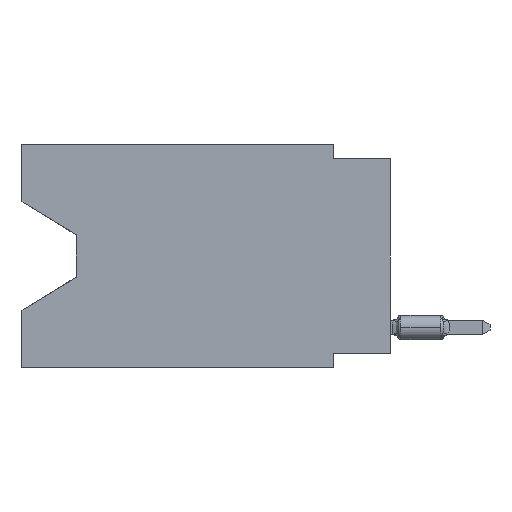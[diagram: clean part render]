
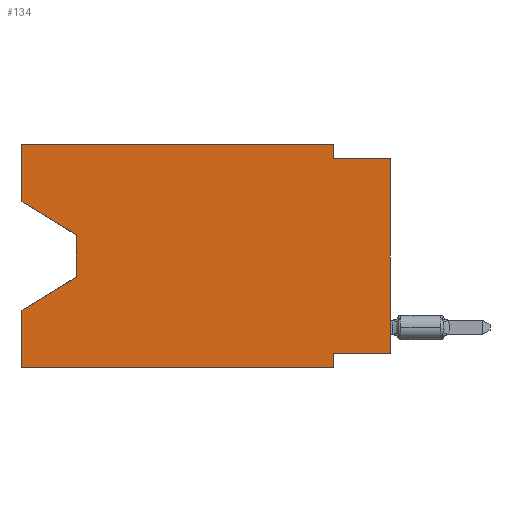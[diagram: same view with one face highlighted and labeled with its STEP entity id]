
A CAD part, left-side view. The second image highlights one B-rep face of the part: STEP entity #134.
In plain terms, the highlighted planar face has unit normal (-1, 0, 0).
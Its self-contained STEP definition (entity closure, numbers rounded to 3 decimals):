
#134 = ADVANCED_FACE ( 'NONE', ( #10927 ), #3493, .F. ) ;
#347 = LINE ( 'NONE', #12735, #4989 ) ;
#407 = LINE ( 'NONE', #6178, #16568 ) ;
#607 = CARTESIAN_POINT ( 'NONE',  ( 0., 2.54, -0.635 ) ) ;
#656 = VECTOR ( 'NONE', #1703, 1000. ) ;
#1014 = CARTESIAN_POINT ( 'NONE',  ( 0., 13.97, -4.013 ) ) ;
#1512 = LINE ( 'NONE', #7038, #6658 ) ;
#1613 = CARTESIAN_POINT ( 'NONE',  ( 0., 16.383, -2.546 ) ) ;
#1703 = DIRECTION ( 'NONE',  ( 0., -1., 0. ) ) ;
#2876 = EDGE_CURVE ( 'NONE', #12312, #13127, #347, .T. ) ;
#3388 = VECTOR ( 'NONE', #4593, 1000. ) ;
#3493 = PLANE ( 'NONE',  #19131 ) ;
#3496 = VERTEX_POINT ( 'NONE', #12833 ) ;
#3534 = ORIENTED_EDGE ( 'NONE', *, *, #12968, .F. ) ;
#3618 = CARTESIAN_POINT ( 'NONE',  ( 0., 16.383, 0. ) ) ;
#3664 = ORIENTED_EDGE ( 'NONE', *, *, #5299, .F. ) ;
#3716 = DIRECTION ( 'NONE',  ( 0., 0., -1. ) ) ;
#3749 = VERTEX_POINT ( 'NONE', #14147 ) ;
#3884 = LINE ( 'NONE', #1613, #22900 ) ;
#3914 = DIRECTION ( 'NONE',  ( 0., 1., 0. ) ) ;
#3937 = EDGE_CURVE ( 'NONE', #19255, #10933, #11486, .T. ) ;
#4223 = CARTESIAN_POINT ( 'NONE',  ( 0., 2.54, -9.906 ) ) ;
#4327 = CARTESIAN_POINT ( 'NONE',  ( 0., 16.383, -2.546 ) ) ;
#4554 = VERTEX_POINT ( 'NONE', #8674 ) ;
#4593 = DIRECTION ( 'NONE',  ( 0., -1., 0. ) ) ;
#4989 = VECTOR ( 'NONE', #3716, 1000. ) ;
#5181 = LINE ( 'NONE', #17962, #12593 ) ;
#5299 = EDGE_CURVE ( 'NONE', #13127, #3749, #19001, .T. ) ;
#6178 = CARTESIAN_POINT ( 'NONE',  ( 0., 16.383, 0. ) ) ;
#6658 = VECTOR ( 'NONE', #21821, 1000. ) ;
#6997 = DIRECTION ( 'NONE',  ( 0., 0., 1. ) ) ;
#7000 = LINE ( 'NONE', #3618, #656 ) ;
#7038 = CARTESIAN_POINT ( 'NONE',  ( 0., 2.54, -9.906 ) ) ;
#7226 = VECTOR ( 'NONE', #3914, 1000. ) ;
#7265 = DIRECTION ( 'NONE',  ( 0., -0.855, -0.519 ) ) ;
#7626 = ORIENTED_EDGE ( 'NONE', *, *, #13353, .T. ) ;
#7737 = DIRECTION ( 'NONE',  ( 0., 0., 1. ) ) ;
#7850 = EDGE_CURVE ( 'NONE', #10156, #19255, #3884, .T. ) ;
#7934 = CARTESIAN_POINT ( 'NONE',  ( 0., 13.97, -5.893 ) ) ;
#8460 = ORIENTED_EDGE ( 'NONE', *, *, #11576, .T. ) ;
#8525 = CARTESIAN_POINT ( 'NONE',  ( 0., 13.97, -5.893 ) ) ;
#8674 = CARTESIAN_POINT ( 'NONE',  ( 0., 16.383, -9.906 ) ) ;
#8904 = ORIENTED_EDGE ( 'NONE', *, *, #2876, .F. ) ;
#9022 = CARTESIAN_POINT ( 'NONE',  ( 0., 16.383, 0. ) ) ;
#9050 = EDGE_CURVE ( 'NONE', #20871, #3749, #5181, .T. ) ;
#9138 = DIRECTION ( 'NONE',  ( 0., 0., -1. ) ) ;
#9290 = EDGE_CURVE ( 'NONE', #20871, #14125, #13063, .T. ) ;
#9650 = CARTESIAN_POINT ( 'NONE',  ( 0., 16.383, -9.906 ) ) ;
#10156 = VERTEX_POINT ( 'NONE', #4327 ) ;
#10237 = VERTEX_POINT ( 'NONE', #4223 ) ;
#10339 = LINE ( 'NONE', #8525, #14000 ) ;
#10630 = EDGE_CURVE ( 'NONE', #3496, #12312, #7000, .T. ) ;
#10927 = FACE_OUTER_BOUND ( 'NONE', #12824, .T. ) ;
#10933 = VERTEX_POINT ( 'NONE', #7934 ) ;
#10942 = DIRECTION ( 'NONE',  ( 0., 0., 1. ) ) ;
#11021 = CARTESIAN_POINT ( 'NONE',  ( 0., 0., -9.271 ) ) ;
#11182 = LINE ( 'NONE', #9022, #15515 ) ;
#11457 = LINE ( 'NONE', #9650, #3388 ) ;
#11486 = LINE ( 'NONE', #1014, #23252 ) ;
#11576 = EDGE_CURVE ( 'NONE', #4554, #10237, #11457, .T. ) ;
#11587 = ORIENTED_EDGE ( 'NONE', *, *, #7850, .T. ) ;
#12312 = VERTEX_POINT ( 'NONE', #16343 ) ;
#12426 = ORIENTED_EDGE ( 'NONE', *, *, #19642, .F. ) ;
#12593 = VECTOR ( 'NONE', #6997, 1000. ) ;
#12735 = CARTESIAN_POINT ( 'NONE',  ( 0., 2.54, 0. ) ) ;
#12824 = EDGE_LOOP ( 'NONE', ( #11587, #17060, #7626, #12426, #8460, #18810, #23030, #22428, #3664, #8904, #22182, #3534 ) ) ;
#12833 = CARTESIAN_POINT ( 'NONE',  ( 0., 16.383, 0. ) ) ;
#12968 = EDGE_CURVE ( 'NONE', #10156, #3496, #11182, .T. ) ;
#13063 = LINE ( 'NONE', #11021, #7226 ) ;
#13127 = VERTEX_POINT ( 'NONE', #607 ) ;
#13335 = DIRECTION ( 'NONE',  ( 0., -1., 0. ) ) ;
#13353 = EDGE_CURVE ( 'NONE', #10933, #22955, #10339, .T. ) ;
#14000 = VECTOR ( 'NONE', #15865, 1000. ) ;
#14125 = VERTEX_POINT ( 'NONE', #17637 ) ;
#14147 = CARTESIAN_POINT ( 'NONE',  ( 0., 0., -0.635 ) ) ;
#14298 = DIRECTION ( 'NONE',  ( 1., 0., 0. ) ) ;
#14894 = EDGE_CURVE ( 'NONE', #14125, #10237, #1512, .T. ) ;
#15515 = VECTOR ( 'NONE', #10942, 1000. ) ;
#15865 = DIRECTION ( 'NONE',  ( 0., 0.855, -0.519 ) ) ;
#16343 = CARTESIAN_POINT ( 'NONE',  ( 0., 2.54, 0. ) ) ;
#16382 = VECTOR ( 'NONE', #13335, 1000. ) ;
#16568 = VECTOR ( 'NONE', #7737, 1000. ) ;
#17060 = ORIENTED_EDGE ( 'NONE', *, *, #3937, .T. ) ;
#17404 = CARTESIAN_POINT ( 'NONE',  ( 0., 13.97, -4.013 ) ) ;
#17430 = CARTESIAN_POINT ( 'NONE',  ( 0., 0., -0.635 ) ) ;
#17637 = CARTESIAN_POINT ( 'NONE',  ( 0., 2.54, -9.271 ) ) ;
#17962 = CARTESIAN_POINT ( 'NONE',  ( 0., 0., 0. ) ) ;
#18810 = ORIENTED_EDGE ( 'NONE', *, *, #14894, .F. ) ;
#18828 = CARTESIAN_POINT ( 'NONE',  ( 0., 0., -9.271 ) ) ;
#19001 = LINE ( 'NONE', #17430, #16382 ) ;
#19131 = AXIS2_PLACEMENT_3D ( 'NONE', #19724, #14298, #9138 ) ;
#19204 = DIRECTION ( 'NONE',  ( 0., 0., -1. ) ) ;
#19255 = VERTEX_POINT ( 'NONE', #17404 ) ;
#19642 = EDGE_CURVE ( 'NONE', #4554, #22955, #407, .T. ) ;
#19724 = CARTESIAN_POINT ( 'NONE',  ( 0., 16.383, 0. ) ) ;
#20193 = CARTESIAN_POINT ( 'NONE',  ( 0., 16.383, -7.36 ) ) ;
#20871 = VERTEX_POINT ( 'NONE', #18828 ) ;
#21821 = DIRECTION ( 'NONE',  ( 0., 0., -1. ) ) ;
#22182 = ORIENTED_EDGE ( 'NONE', *, *, #10630, .F. ) ;
#22428 = ORIENTED_EDGE ( 'NONE', *, *, #9050, .T. ) ;
#22900 = VECTOR ( 'NONE', #7265, 1000. ) ;
#22955 = VERTEX_POINT ( 'NONE', #20193 ) ;
#23030 = ORIENTED_EDGE ( 'NONE', *, *, #9290, .F. ) ;
#23252 = VECTOR ( 'NONE', #19204, 1000. ) ;
